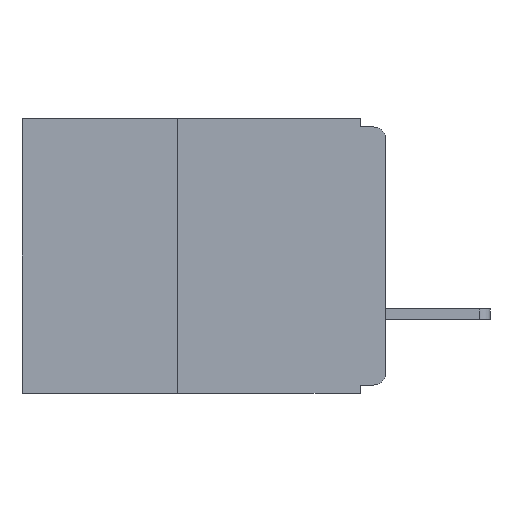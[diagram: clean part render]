
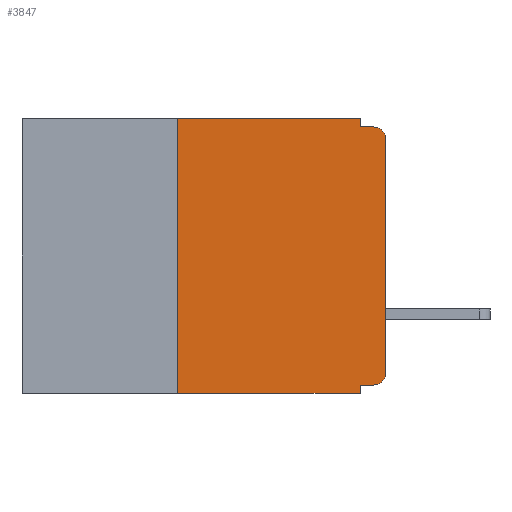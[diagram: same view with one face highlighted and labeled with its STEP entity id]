
A CAD part, left-side view. The second image highlights one B-rep face of the part: STEP entity #3847.
In plain terms, the highlighted planar face has unit normal (-1, 0, 0).
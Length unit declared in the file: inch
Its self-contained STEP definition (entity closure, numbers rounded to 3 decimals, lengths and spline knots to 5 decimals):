
#275 = VERTEX_POINT ( 'NONE', #2039 ) ;
#430 = DIRECTION ( 'NONE',  ( 1., 0., 0. ) ) ;
#714 = DIRECTION ( 'NONE',  ( -1., 0., 0. ) ) ;
#867 = VECTOR ( 'NONE', #6420, 39.37008 ) ;
#913 = VERTEX_POINT ( 'NONE', #3861 ) ;
#1952 = CARTESIAN_POINT ( 'NONE',  ( 0., 0.015, -0.32 ) ) ;
#2039 = CARTESIAN_POINT ( 'NONE',  ( 0., 0.25, -0.33 ) ) ;
#2078 = CARTESIAN_POINT ( 'NONE',  ( 0., 0.437, 0. ) ) ;
#2217 = CARTESIAN_POINT ( 'NONE',  ( 0., 0.031, 0. ) ) ;
#2471 = CIRCLE ( 'NONE', #8571, 0.015 ) ;
#2827 = DIRECTION ( 'NONE',  ( 0., 0., 1. ) ) ;
#2910 = ORIENTED_EDGE ( 'NONE', *, *, #7167, .T. ) ;
#3015 = ORIENTED_EDGE ( 'NONE', *, *, #3334, .T. ) ;
#3075 = VERTEX_POINT ( 'NONE', #6906 ) ;
#3179 = VERTEX_POINT ( 'NONE', #1952 ) ;
#3334 = EDGE_CURVE ( 'NONE', #913, #11793, #2471, .T. ) ;
#3436 = CARTESIAN_POINT ( 'NONE',  ( 0., 0.031, -0.32 ) ) ;
#3847 = ADVANCED_FACE ( 'NONE', ( #9935 ), #8991, .F. ) ;
#3861 = CARTESIAN_POINT ( 'NONE',  ( 0., 0., -0.025 ) ) ;
#4322 = CIRCLE ( 'NONE', #5539, 0.015 ) ;
#4541 = ORIENTED_EDGE ( 'NONE', *, *, #14595, .F. ) ;
#4649 = CARTESIAN_POINT ( 'NONE',  ( 0., 0.031, -0.33 ) ) ;
#5091 = ORIENTED_EDGE ( 'NONE', *, *, #14757, .T. ) ;
#5210 = CARTESIAN_POINT ( 'NONE',  ( 0., 0., 0. ) ) ;
#5260 = CARTESIAN_POINT ( 'NONE',  ( 0., 0.031, -0.33 ) ) ;
#5461 = CARTESIAN_POINT ( 'NONE',  ( 0., 0., -0.32 ) ) ;
#5539 = AXIS2_PLACEMENT_3D ( 'NONE', #10954, #714, #12618 ) ;
#5622 = ORIENTED_EDGE ( 'NONE', *, *, #9942, .F. ) ;
#6014 = LINE ( 'NONE', #12120, #10463 ) ;
#6243 = CARTESIAN_POINT ( 'NONE',  ( 0., 0.031, -0.01 ) ) ;
#6420 = DIRECTION ( 'NONE',  ( 0., 0., -1. ) ) ;
#6497 = CARTESIAN_POINT ( 'NONE',  ( 0., 0.25, 0. ) ) ;
#6906 = CARTESIAN_POINT ( 'NONE',  ( 0., 0., -0.305 ) ) ;
#6930 = VERTEX_POINT ( 'NONE', #3436 ) ;
#7167 = EDGE_CURVE ( 'NONE', #3179, #3075, #4322, .T. ) ;
#7464 = DIRECTION ( 'NONE',  ( 0., 0., -1. ) ) ;
#7648 = CARTESIAN_POINT ( 'NONE',  ( 0., 0.015, -0.025 ) ) ;
#7745 = AXIS2_PLACEMENT_3D ( 'NONE', #2078, #430, #12340 ) ;
#8571 = AXIS2_PLACEMENT_3D ( 'NONE', #7648, #19219, #9306 ) ;
#8991 = PLANE ( 'NONE',  #7745 ) ;
#9306 = DIRECTION ( 'NONE',  ( 0., 0., -1. ) ) ;
#9327 = ORIENTED_EDGE ( 'NONE', *, *, #12547, .F. ) ;
#9527 = LINE ( 'NONE', #2217, #13434 ) ;
#9798 = LINE ( 'NONE', #5461, #13702 ) ;
#9935 = FACE_OUTER_BOUND ( 'NONE', #13295, .T. ) ;
#9942 = EDGE_CURVE ( 'NONE', #20366, #14005, #9527, .T. ) ;
#10463 = VECTOR ( 'NONE', #13799, 39.37008 ) ;
#10875 = CARTESIAN_POINT ( 'NONE',  ( 0., 0., -0.01 ) ) ;
#10954 = CARTESIAN_POINT ( 'NONE',  ( 0., 0.015, -0.305 ) ) ;
#11140 = ORIENTED_EDGE ( 'NONE', *, *, #17103, .F. ) ;
#11300 = LINE ( 'NONE', #10875, #20045 ) ;
#11715 = DIRECTION ( 'NONE',  ( 0., -1., 0. ) ) ;
#11793 = VERTEX_POINT ( 'NONE', #11805 ) ;
#11805 = CARTESIAN_POINT ( 'NONE',  ( 0., 0.015, -0.01 ) ) ;
#12120 = CARTESIAN_POINT ( 'NONE',  ( 0., 0.437, 0. ) ) ;
#12340 = DIRECTION ( 'NONE',  ( 0., 0., -1. ) ) ;
#12547 = EDGE_CURVE ( 'NONE', #3179, #6930, #9798, .T. ) ;
#12618 = DIRECTION ( 'NONE',  ( 0., 0., -1. ) ) ;
#13295 = EDGE_LOOP ( 'NONE', ( #17229, #3015, #15833, #5622, #20902, #4541, #5091, #11140, #9327, #2910 ) ) ;
#13434 = VECTOR ( 'NONE', #7464, 39.37008 ) ;
#13702 = VECTOR ( 'NONE', #17153, 39.37008 ) ;
#13799 = DIRECTION ( 'NONE',  ( 0., -1., 0. ) ) ;
#14005 = VERTEX_POINT ( 'NONE', #6243 ) ;
#14404 = EDGE_CURVE ( 'NONE', #14005, #11793, #11300, .T. ) ;
#14433 = LINE ( 'NONE', #4649, #867 ) ;
#14595 = EDGE_CURVE ( 'NONE', #275, #17128, #15986, .T. ) ;
#14757 = EDGE_CURVE ( 'NONE', #275, #18982, #17260, .T. ) ;
#14860 = VECTOR ( 'NONE', #16990, 39.37008 ) ;
#15522 = EDGE_CURVE ( 'NONE', #17128, #20366, #6014, .T. ) ;
#15833 = ORIENTED_EDGE ( 'NONE', *, *, #14404, .F. ) ;
#15986 = LINE ( 'NONE', #21180, #20285 ) ;
#16747 = VECTOR ( 'NONE', #11715, 39.37008 ) ;
#16990 = DIRECTION ( 'NONE',  ( 0., 0., 1. ) ) ;
#17103 = EDGE_CURVE ( 'NONE', #6930, #18982, #14433, .T. ) ;
#17128 = VERTEX_POINT ( 'NONE', #6497 ) ;
#17153 = DIRECTION ( 'NONE',  ( 0., 1., 0. ) ) ;
#17229 = ORIENTED_EDGE ( 'NONE', *, *, #19842, .T. ) ;
#17260 = LINE ( 'NONE', #21522, #16747 ) ;
#18982 = VERTEX_POINT ( 'NONE', #5260 ) ;
#19117 = DIRECTION ( 'NONE',  ( 0., -1., 0. ) ) ;
#19204 = LINE ( 'NONE', #5210, #14860 ) ;
#19219 = DIRECTION ( 'NONE',  ( -1., 0., 0. ) ) ;
#19842 = EDGE_CURVE ( 'NONE', #3075, #913, #19204, .T. ) ;
#20045 = VECTOR ( 'NONE', #19117, 39.37008 ) ;
#20285 = VECTOR ( 'NONE', #2827, 39.37008 ) ;
#20366 = VERTEX_POINT ( 'NONE', #21463 ) ;
#20902 = ORIENTED_EDGE ( 'NONE', *, *, #15522, .F. ) ;
#21180 = CARTESIAN_POINT ( 'NONE',  ( 0., 0.25, -0.33 ) ) ;
#21463 = CARTESIAN_POINT ( 'NONE',  ( 0., 0.031, 0. ) ) ;
#21522 = CARTESIAN_POINT ( 'NONE',  ( 0., 0.437, -0.33 ) ) ;
